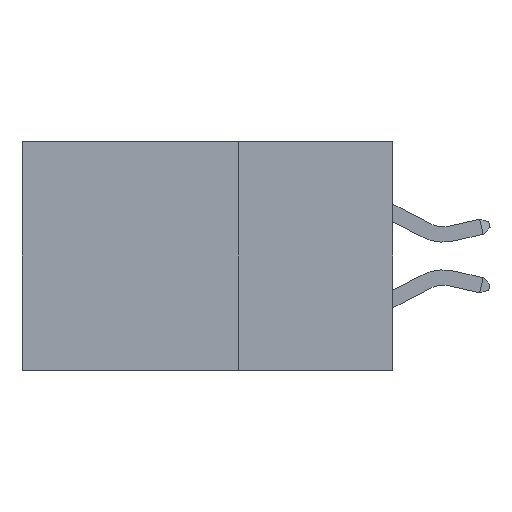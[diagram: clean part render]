
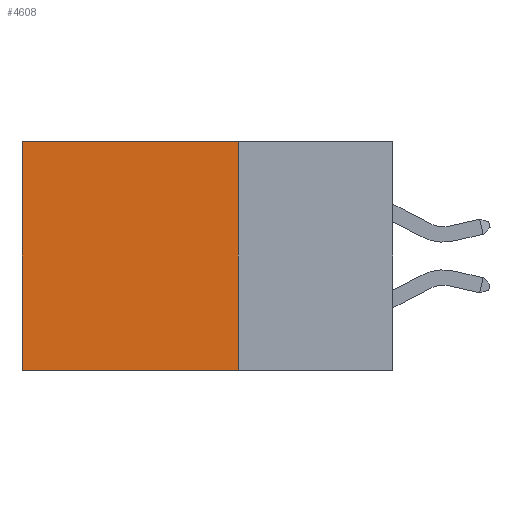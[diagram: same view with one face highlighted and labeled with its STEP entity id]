
A CAD part, left-side view. The second image highlights one B-rep face of the part: STEP entity #4608.
In plain terms, the highlighted planar face has unit normal (-1, 0, 0).
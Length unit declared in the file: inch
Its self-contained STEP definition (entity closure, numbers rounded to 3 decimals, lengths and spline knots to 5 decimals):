
#914 = DIRECTION ( 'NONE',  ( 0., 0., -1. ) ) ;
#1091 = VERTEX_POINT ( 'NONE', #3011 ) ;
#2384 = EDGE_CURVE ( 'NONE', #25268, #37761, #9181, .T. ) ;
#3011 = CARTESIAN_POINT ( 'NONE',  ( 0.2875, 0.6, -0.37 ) ) ;
#3167 = CARTESIAN_POINT ( 'NONE',  ( 0.2875, 0.25, 0. ) ) ;
#3843 = CARTESIAN_POINT ( 'NONE',  ( 0.2875, 0.25, 0. ) ) ;
#4608 = ADVANCED_FACE ( 'NONE', ( #5092 ), #15373, .F. ) ;
#5092 = FACE_OUTER_BOUND ( 'NONE', #34863, .T. ) ;
#7315 = LINE ( 'NONE', #13621, #27817 ) ;
#8873 = DIRECTION ( 'NONE',  ( 0., 0., -1. ) ) ;
#8911 = ORIENTED_EDGE ( 'NONE', *, *, #2384, .T. ) ;
#9181 = LINE ( 'NONE', #27839, #26268 ) ;
#9622 = VECTOR ( 'NONE', #13239, 39.37008 ) ;
#10283 = CARTESIAN_POINT ( 'NONE',  ( 0.2875, 0.25, -0.37 ) ) ;
#11398 = CARTESIAN_POINT ( 'NONE',  ( 0.2875, 0.25, 0. ) ) ;
#13034 = ORIENTED_EDGE ( 'NONE', *, *, #32787, .T. ) ;
#13239 = DIRECTION ( 'NONE',  ( 0., 1., 0. ) ) ;
#13621 = CARTESIAN_POINT ( 'NONE',  ( 0.2875, 0.6, 0. ) ) ;
#15159 = EDGE_CURVE ( 'NONE', #25268, #16284, #33408, .T. ) ;
#15165 = DIRECTION ( 'NONE',  ( 1., 0., 0. ) ) ;
#15373 = PLANE ( 'NONE',  #26474 ) ;
#16284 = VERTEX_POINT ( 'NONE', #35175 ) ;
#21963 = DIRECTION ( 'NONE',  ( 0., 1., 0. ) ) ;
#23751 = ORIENTED_EDGE ( 'NONE', *, *, #15159, .F. ) ;
#25268 = VERTEX_POINT ( 'NONE', #3167 ) ;
#25463 = EDGE_CURVE ( 'NONE', #16284, #1091, #26220, .T. ) ;
#26220 = LINE ( 'NONE', #10283, #9622 ) ;
#26268 = VECTOR ( 'NONE', #21963, 39.37008 ) ;
#26474 = AXIS2_PLACEMENT_3D ( 'NONE', #11398, #15165, #8873 ) ;
#27817 = VECTOR ( 'NONE', #31896, 39.37008 ) ;
#27839 = CARTESIAN_POINT ( 'NONE',  ( 0.2875, 0.25, 0. ) ) ;
#31896 = DIRECTION ( 'NONE',  ( 0., 0., -1. ) ) ;
#32787 = EDGE_CURVE ( 'NONE', #37761, #1091, #7315, .T. ) ;
#33408 = LINE ( 'NONE', #3843, #38685 ) ;
#34735 = CARTESIAN_POINT ( 'NONE',  ( 0.2875, 0.6, 0. ) ) ;
#34863 = EDGE_LOOP ( 'NONE', ( #13034, #36320, #23751, #8911 ) ) ;
#35175 = CARTESIAN_POINT ( 'NONE',  ( 0.2875, 0.25, -0.37 ) ) ;
#36320 = ORIENTED_EDGE ( 'NONE', *, *, #25463, .F. ) ;
#37761 = VERTEX_POINT ( 'NONE', #34735 ) ;
#38685 = VECTOR ( 'NONE', #914, 39.37008 ) ;
